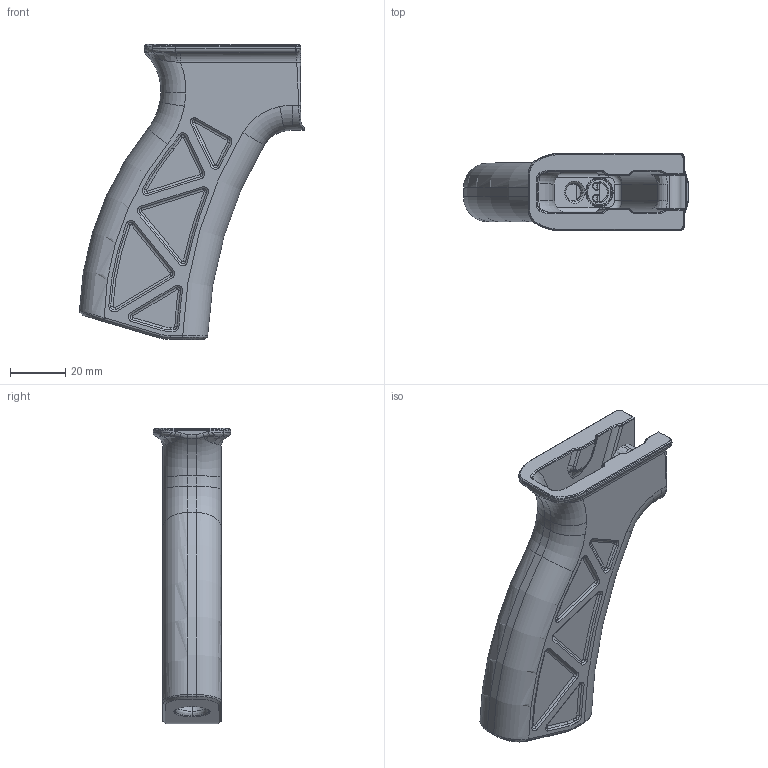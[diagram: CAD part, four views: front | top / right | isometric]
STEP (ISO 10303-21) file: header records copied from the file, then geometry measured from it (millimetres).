
FILE_DESCRIPTION(/* description */ (''),/* implementation_level */ '2;1');
FILE_NAME(/* name */ 'Tri Indent Grip.step',/* time_stamp */ '2021-09-20T01:27:25-04:00',/* author */ (''),/* organization */ (''),/* preprocessor_version */ 'ST-DEVELOPER v18.1',/* originating_system */ 'Autodesk Translation Framework v10.10.0.1391',/* authorisation */ '');
FILE_SCHEMA (('AUTOMOTIVE_DESIGN { 1 0 10303 214 3 1 1 }'));
Length unit declared in the file: millimetre
Products named in the file (1): Tri Indent Grip
Bounding box: 81.2 x 28 x 106.49 mm (x, y, z)
Volume: 50560.1 mm3; surface area: 25718.3 mm2
Topology: 1 solids, 1 shells, 600 faces, 1432 edges, 840 vertices
Faces by surface type: bspline 270, cylinder 125, plane 84, torus 71, cone 50
Entity records: 23020 total; most frequent: CARTESIAN_POINT 10489, ORIENTED_EDGE 2840, DIRECTION 2239, EDGE_CURVE 1420, AXIS2_PLACEMENT_3D 921, VERTEX_POINT 840, EDGE_LOOP 620, FACE_OUTER_BOUND 600
